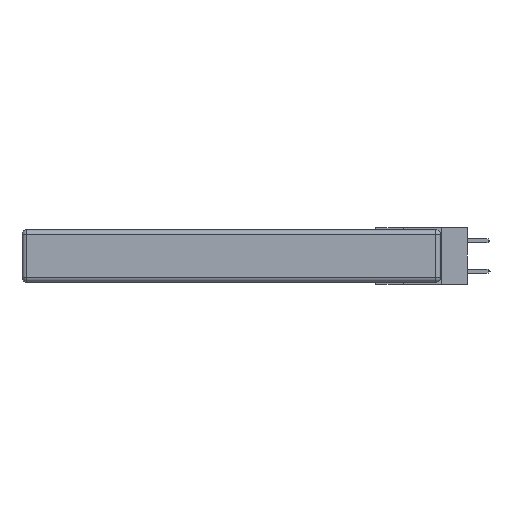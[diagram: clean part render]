
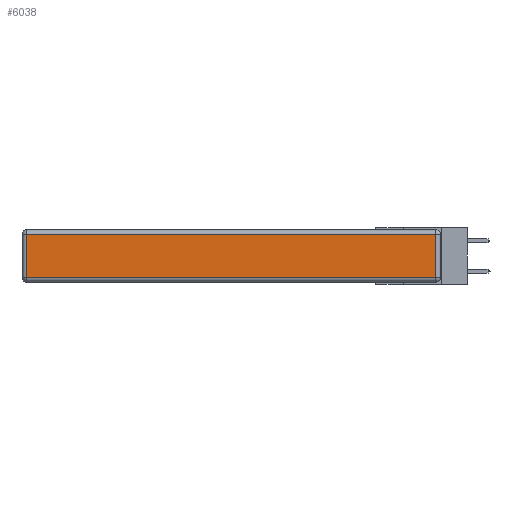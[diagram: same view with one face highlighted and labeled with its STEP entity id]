
A CAD part, left-side view. The second image highlights one B-rep face of the part: STEP entity #6038.
In plain terms, the highlighted planar face has unit normal (-1, 0, 0).
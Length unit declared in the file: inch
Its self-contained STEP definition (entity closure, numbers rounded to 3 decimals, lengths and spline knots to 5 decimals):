
#27 = VERTEX_POINT ( 'NONE', #5106 ) ;
#205 = DIRECTION ( 'NONE',  ( -1., 0., 0. ) ) ;
#344 = DIRECTION ( 'NONE',  ( 0., 0., 1. ) ) ;
#367 = LINE ( 'NONE', #2559, #12195 ) ;
#835 = VECTOR ( 'NONE', #11363, 39.37008 ) ;
#1112 = VERTEX_POINT ( 'NONE', #5419 ) ;
#1288 = ORIENTED_EDGE ( 'NONE', *, *, #3411, .T. ) ;
#1340 = VECTOR ( 'NONE', #344, 39.37008 ) ;
#2132 = DIRECTION ( 'NONE',  ( 0., 0., 1. ) ) ;
#2559 = CARTESIAN_POINT ( 'NONE',  ( 0., 2.75, -0.03 ) ) ;
#2809 = CARTESIAN_POINT ( 'NONE',  ( 0., 2.72, -0.343 ) ) ;
#2813 = CARTESIAN_POINT ( 'NONE',  ( 0., 2.72, -0.313 ) ) ;
#3336 = LINE ( 'NONE', #2809, #835 ) ;
#3411 = EDGE_CURVE ( 'NONE', #5067, #27, #367, .T. ) ;
#4518 = VERTEX_POINT ( 'NONE', #2813 ) ;
#4670 = CARTESIAN_POINT ( 'NONE',  ( 0., 0., -0.313 ) ) ;
#5067 = VERTEX_POINT ( 'NONE', #5239 ) ;
#5106 = CARTESIAN_POINT ( 'NONE',  ( 0., 2.72, -0.03 ) ) ;
#5239 = CARTESIAN_POINT ( 'NONE',  ( 0., 0.03, -0.03 ) ) ;
#5419 = CARTESIAN_POINT ( 'NONE',  ( 0., 0.03, -0.313 ) ) ;
#5577 = DIRECTION ( 'NONE',  ( 0., -1., 0. ) ) ;
#5856 = CARTESIAN_POINT ( 'NONE',  ( 0., 0., -0.343 ) ) ;
#6038 = ADVANCED_FACE ( 'NONE', ( #11561 ), #6846, .T. ) ;
#6305 = EDGE_CURVE ( 'NONE', #1112, #5067, #7824, .T. ) ;
#6846 = PLANE ( 'NONE',  #9255 ) ;
#7031 = EDGE_CURVE ( 'NONE', #4518, #1112, #9304, .T. ) ;
#7350 = DIRECTION ( 'NONE',  ( 0., 1., 0. ) ) ;
#7809 = ORIENTED_EDGE ( 'NONE', *, *, #11514, .T. ) ;
#7818 = EDGE_LOOP ( 'NONE', ( #11307, #9049, #1288, #7809 ) ) ;
#7824 = LINE ( 'NONE', #11601, #1340 ) ;
#9049 = ORIENTED_EDGE ( 'NONE', *, *, #6305, .T. ) ;
#9255 = AXIS2_PLACEMENT_3D ( 'NONE', #5856, #205, #2132 ) ;
#9304 = LINE ( 'NONE', #4670, #11846 ) ;
#11307 = ORIENTED_EDGE ( 'NONE', *, *, #7031, .T. ) ;
#11363 = DIRECTION ( 'NONE',  ( 0., 0., -1. ) ) ;
#11514 = EDGE_CURVE ( 'NONE', #27, #4518, #3336, .T. ) ;
#11561 = FACE_OUTER_BOUND ( 'NONE', #7818, .T. ) ;
#11601 = CARTESIAN_POINT ( 'NONE',  ( 0., 0.03, -0.343 ) ) ;
#11846 = VECTOR ( 'NONE', #5577, 39.37008 ) ;
#12195 = VECTOR ( 'NONE', #7350, 39.37008 ) ;
